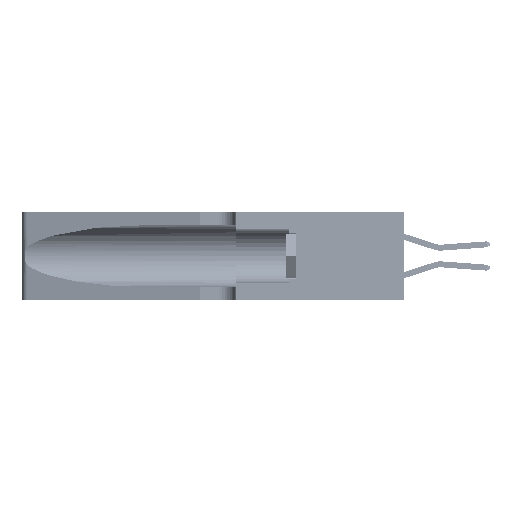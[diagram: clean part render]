
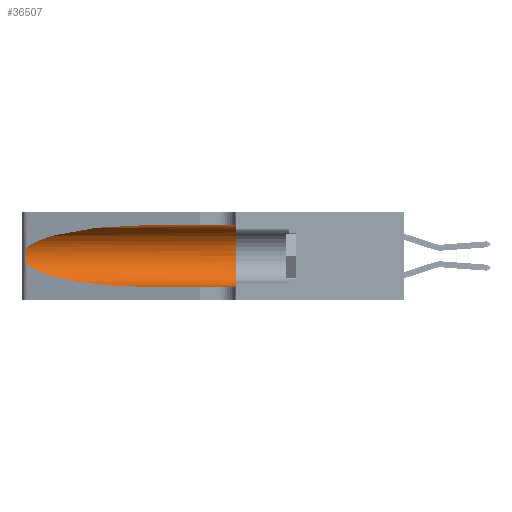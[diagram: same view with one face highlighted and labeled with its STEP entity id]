
A CAD part, left-side view. The second image highlights one B-rep face of the part: STEP entity #36507.
In plain terms, the highlighted cylindrical face has radius 3.308 mm (diameter 6.617 mm), a partial arc.
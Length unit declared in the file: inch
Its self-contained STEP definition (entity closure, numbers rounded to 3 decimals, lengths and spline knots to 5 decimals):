
#1596 = CARTESIAN_POINT ( 'NONE',  ( 0.1305, 1.61858, 0.31525 ) ) ;
#1651 = CARTESIAN_POINT ( 'NONE',  ( 0.25555, 1.22993, 0.14849 ) ) ;
#2922 = CARTESIAN_POINT ( 'NONE',  ( 0.18966, 0.96281, 0.05475 ) ) ;
#3583 = VERTEX_POINT ( 'NONE', #38093 ) ;
#4502 = CARTESIAN_POINT ( 'NONE',  ( 0.1305, 0.72297, 0.31525 ) ) ;
#5818 = DIRECTION ( 'NONE',  ( 0., -1., 0. ) ) ;
#7118 = CARTESIAN_POINT ( 'NONE',  ( 0.25487, 1.22718, 0.14631 ) ) ;
#8306 = CARTESIAN_POINT ( 'NONE',  ( 0.25487, 1.22718, 0.22369 ) ) ;
#8401 = VECTOR ( 'NONE', #47273, 39.37008 ) ;
#8468 = VERTEX_POINT ( 'NONE', #8306 ) ;
#9922 = CARTESIAN_POINT ( 'NONE',  ( 0.25787, 1.23484, 0.2124 ) ) ;
#11469 = AXIS2_PLACEMENT_3D ( 'NONE', #43004, #18321, #47125 ) ;
#13836 = ORIENTED_EDGE ( 'NONE', *, *, #48959, .T. ) ;
#14074 = CARTESIAN_POINT ( 'NONE',  ( 0.26018, 1.23835, 0.19895 ) ) ;
#14127 = VERTEX_POINT ( 'NONE', #7118 ) ;
#14389 = EDGE_CURVE ( 'NONE', #27581, #8468, #41318, .T. ) ;
#14855 = CARTESIAN_POINT ( 'NONE',  ( 0.1305, 1.61858, 0.185 ) ) ;
#17137 = CARTESIAN_POINT ( 'NONE',  ( 0.18966, 0.96281, 0.31525 ) ) ;
#17758 = EDGE_CURVE ( 'NONE', #8468, #14127, #29993, .T. ) ;
#18174 = LINE ( 'NONE', #43144, #8401 ) ;
#18313 = CARTESIAN_POINT ( 'NONE',  ( 0.26075, 1.23896, 0.178 ) ) ;
#18321 = DIRECTION ( 'NONE',  ( 0., 1., 0. ) ) ;
#19107 = LINE ( 'NONE', #1596, #39741 ) ;
#20459 = EDGE_CURVE ( 'NONE', #27581, #42605, #19107, .T. ) ;
#21055 = EDGE_LOOP ( 'NONE', ( #41981, #43867, #13836, #53271, #41685, #48717 ) ) ;
#22374 = CARTESIAN_POINT ( 'NONE',  ( 0.25487, 1.22718, 0.22369 ) ) ;
#22548 = CARTESIAN_POINT ( 'NONE',  ( 0.25856, 1.23593, 0.16098 ) ) ;
#22573 =( BOUNDED_CURVE ( )  B_SPLINE_CURVE ( 3, ( #23774, #52445, #2922, #32026 ),
 .UNSPECIFIED., .F., .F. ) 
 B_SPLINE_CURVE_WITH_KNOTS ( ( 4, 4 ),
 ( 3.44316, 4.71239 ),
 .UNSPECIFIED. ) 
 CURVE ( )  GEOMETRIC_REPRESENTATION_ITEM ( )  RATIONAL_B_SPLINE_CURVE ( ( 1., 0.87, 0.87, 1. ) ) 
 REPRESENTATION_ITEM ( '' )  );
#23774 = CARTESIAN_POINT ( 'NONE',  ( 0.25487, 1.22718, 0.14631 ) ) ;
#24972 = EDGE_CURVE ( 'NONE', #42605, #36798, #33649, .T. ) ;
#25522 = CARTESIAN_POINT ( 'NONE',  ( 0.25487, 1.22718, 0.22369 ) ) ;
#26677 = CARTESIAN_POINT ( 'NONE',  ( 0.25639, 1.23186, 0.15144 ) ) ;
#27581 = VERTEX_POINT ( 'NONE', #46422 ) ;
#29993 = B_SPLINE_CURVE_WITH_KNOTS ( 'NONE', 3,
 ( #22374, #46937, #34761, #9922, #38900, #14074, #42999, #18313, #47120, #22548, #51230, #26677, #1651, #30797 ),
 .UNSPECIFIED., .F., .F.,
 ( 4, 2, 2, 2, 2, 2, 4 ),
 ( 0., 0.00027, 0.00053, 0.00107, 0.0016, 0.00187, 0.00214 ),
 .UNSPECIFIED. ) ;
#30797 = CARTESIAN_POINT ( 'NONE',  ( 0.25487, 1.22718, 0.14631 ) ) ;
#31376 = DIRECTION ( 'NONE',  ( 0., -1., 0. ) ) ;
#32026 = CARTESIAN_POINT ( 'NONE',  ( 0.1305, 0.72297, 0.05475 ) ) ;
#33649 = CIRCLE ( 'NONE', #11469, 0.13025 ) ;
#34761 = CARTESIAN_POINT ( 'NONE',  ( 0.25639, 1.23184, 0.21858 ) ) ;
#36507 = ADVANCED_FACE ( 'NONE', ( #50688 ), #49415, .F. ) ;
#36798 = VERTEX_POINT ( 'NONE', #49296 ) ;
#38093 = CARTESIAN_POINT ( 'NONE',  ( 0.1305, 0.72297, 0.05475 ) ) ;
#38900 = CARTESIAN_POINT ( 'NONE',  ( 0.25854, 1.2359, 0.20912 ) ) ;
#39741 = VECTOR ( 'NONE', #5818, 39.37008 ) ;
#41318 =( BOUNDED_CURVE ( )  B_SPLINE_CURVE ( 3, ( #4502, #17137, #50082, #25522 ),
 .UNSPECIFIED., .F., .F. ) 
 B_SPLINE_CURVE_WITH_KNOTS ( ( 4, 4 ),
 ( 1.5708, 2.84003 ),
 .UNSPECIFIED. ) 
 CURVE ( )  GEOMETRIC_REPRESENTATION_ITEM ( )  RATIONAL_B_SPLINE_CURVE ( ( 1., 0.87, 0.87, 1. ) ) 
 REPRESENTATION_ITEM ( '' )  );
#41685 = ORIENTED_EDGE ( 'NONE', *, *, #24972, .F. ) ;
#41981 = ORIENTED_EDGE ( 'NONE', *, *, #14389, .T. ) ;
#42504 = CARTESIAN_POINT ( 'NONE',  ( 0.1305, 0.35, 0.31525 ) ) ;
#42605 = VERTEX_POINT ( 'NONE', #42504 ) ;
#42999 = CARTESIAN_POINT ( 'NONE',  ( 0.26075, 1.23896, 0.19203 ) ) ;
#43004 = CARTESIAN_POINT ( 'NONE',  ( 0.1305, 0.35, 0.185 ) ) ;
#43144 = CARTESIAN_POINT ( 'NONE',  ( 0.1305, 1.61858, 0.05475 ) ) ;
#43754 = DIRECTION ( 'NONE',  ( 0., 0., -1. ) ) ;
#43867 = ORIENTED_EDGE ( 'NONE', *, *, #17758, .T. ) ;
#44724 = AXIS2_PLACEMENT_3D ( 'NONE', #14855, #31376, #43754 ) ;
#45317 = EDGE_CURVE ( 'NONE', #3583, #36798, #18174, .T. ) ;
#46422 = CARTESIAN_POINT ( 'NONE',  ( 0.1305, 0.72297, 0.31525 ) ) ;
#46937 = CARTESIAN_POINT ( 'NONE',  ( 0.25555, 1.22994, 0.2215 ) ) ;
#47120 = CARTESIAN_POINT ( 'NONE',  ( 0.26017, 1.23833, 0.17102 ) ) ;
#47125 = DIRECTION ( 'NONE',  ( 0., 0., 1. ) ) ;
#47273 = DIRECTION ( 'NONE',  ( 0., -1., 0. ) ) ;
#48717 = ORIENTED_EDGE ( 'NONE', *, *, #20459, .F. ) ;
#48959 = EDGE_CURVE ( 'NONE', #14127, #3583, #22573, .T. ) ;
#49296 = CARTESIAN_POINT ( 'NONE',  ( 0.1305, 0.35, 0.05475 ) ) ;
#49415 = CYLINDRICAL_SURFACE ( 'NONE', #44724, 0.13025 ) ;
#50082 = CARTESIAN_POINT ( 'NONE',  ( 0.2373, 1.15595, 0.28018 ) ) ;
#50688 = FACE_OUTER_BOUND ( 'NONE', #21055, .T. ) ;
#51230 = CARTESIAN_POINT ( 'NONE',  ( 0.25789, 1.23486, 0.15765 ) ) ;
#52445 = CARTESIAN_POINT ( 'NONE',  ( 0.2373, 1.15595, 0.08982 ) ) ;
#53271 = ORIENTED_EDGE ( 'NONE', *, *, #45317, .T. ) ;
